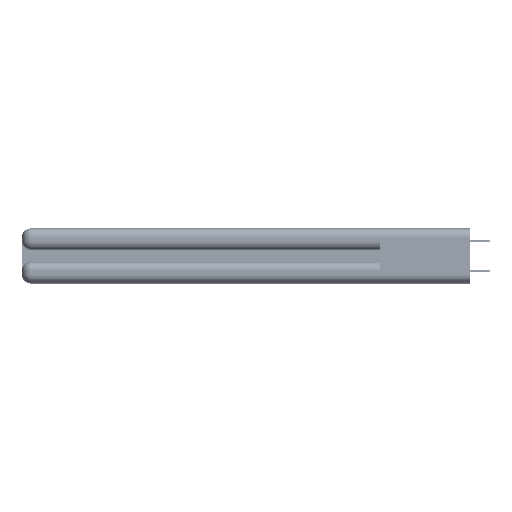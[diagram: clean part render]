
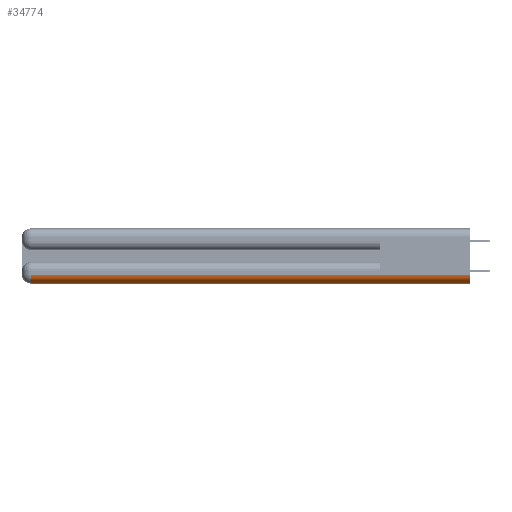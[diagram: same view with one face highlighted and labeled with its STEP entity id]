
A CAD part, left-side view. The second image highlights one B-rep face of the part: STEP entity #34774.
In plain terms, the highlighted cylindrical face has radius 1.524 mm (diameter 3.048 mm), a partial arc.
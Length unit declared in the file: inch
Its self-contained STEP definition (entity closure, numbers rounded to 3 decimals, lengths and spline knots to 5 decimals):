
#213 = EDGE_CURVE ( 'NONE', #34212, #19637, #16838, .T. ) ;
#2609 = VECTOR ( 'NONE', #23234, 39.37008 ) ;
#4118 = CYLINDRICAL_SURFACE ( 'NONE', #52837, 0.06 ) ;
#4308 = VERTEX_POINT ( 'NONE', #30199 ) ;
#7576 = ORIENTED_EDGE ( 'NONE', *, *, #19546, .F. ) ;
#8139 = EDGE_CURVE ( 'NONE', #27237, #34212, #28561, .T. ) ;
#13064 = ORIENTED_EDGE ( 'NONE', *, *, #21346, .F. ) ;
#15577 = ORIENTED_EDGE ( 'NONE', *, *, #8139, .F. ) ;
#16037 = EDGE_LOOP ( 'NONE', ( #13064, #37710, #15577, #7576 ) ) ;
#16838 = LINE ( 'NONE', #20433, #28580 ) ;
#17075 = DIRECTION ( 'NONE',  ( 0., 0., 1. ) ) ;
#19112 = CARTESIAN_POINT ( 'NONE',  ( 0.06, 3., 0. ) ) ;
#19381 = LINE ( 'NONE', #19112, #2609 ) ;
#19546 = EDGE_CURVE ( 'NONE', #4308, #27237, #19381, .T. ) ;
#19637 = VERTEX_POINT ( 'NONE', #41632 ) ;
#20127 = DIRECTION ( 'NONE',  ( 0., 0., 1. ) ) ;
#20433 = CARTESIAN_POINT ( 'NONE',  ( 0., 0., 0.06 ) ) ;
#21346 = EDGE_CURVE ( 'NONE', #19637, #4308, #27288, .T. ) ;
#23234 = DIRECTION ( 'NONE',  ( 0., 1., 0. ) ) ;
#24891 = CARTESIAN_POINT ( 'NONE',  ( 0.06, 2.94, 0.06 ) ) ;
#25393 = DIRECTION ( 'NONE',  ( 0., -1., 0. ) ) ;
#27237 = VERTEX_POINT ( 'NONE', #44830 ) ;
#27288 = CIRCLE ( 'NONE', #53696, 0.06 ) ;
#28561 = CIRCLE ( 'NONE', #32120, 0.06 ) ;
#28580 = VECTOR ( 'NONE', #25393, 39.37008 ) ;
#29838 = DIRECTION ( 'NONE',  ( 0., 0., 1. ) ) ;
#30199 = CARTESIAN_POINT ( 'NONE',  ( 0.06, 0., 0. ) ) ;
#32120 = AXIS2_PLACEMENT_3D ( 'NONE', #24891, #42491, #29838 ) ;
#34212 = VERTEX_POINT ( 'NONE', #42477 ) ;
#34774 = ADVANCED_FACE ( 'NONE', ( #41866 ), #4118, .T. ) ;
#37710 = ORIENTED_EDGE ( 'NONE', *, *, #213, .F. ) ;
#41632 = CARTESIAN_POINT ( 'NONE',  ( 0., 0., 0.06 ) ) ;
#41866 = FACE_OUTER_BOUND ( 'NONE', #16037, .T. ) ;
#42124 = DIRECTION ( 'NONE',  ( 0., -1., 0. ) ) ;
#42137 = CARTESIAN_POINT ( 'NONE',  ( 0.06, 0., 0.06 ) ) ;
#42477 = CARTESIAN_POINT ( 'NONE',  ( 0., 2.94, 0.06 ) ) ;
#42491 = DIRECTION ( 'NONE',  ( 0., 1., 0. ) ) ;
#44830 = CARTESIAN_POINT ( 'NONE',  ( 0.06, 2.94, 0. ) ) ;
#45998 = CARTESIAN_POINT ( 'NONE',  ( 0.06, 0., 0.06 ) ) ;
#50146 = DIRECTION ( 'NONE',  ( 0., 1., 0. ) ) ;
#52837 = AXIS2_PLACEMENT_3D ( 'NONE', #42137, #50146, #17075 ) ;
#53696 = AXIS2_PLACEMENT_3D ( 'NONE', #45998, #42124, #20127 ) ;
